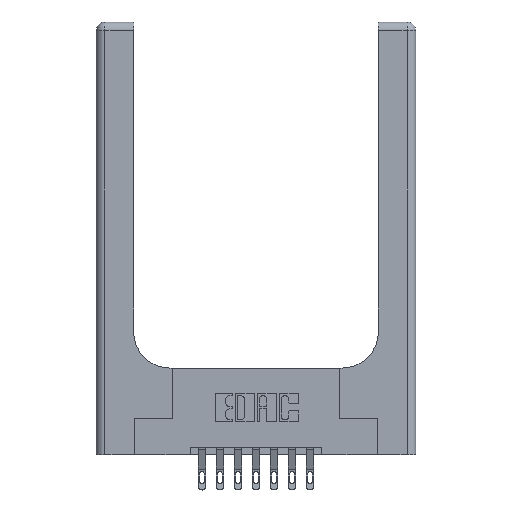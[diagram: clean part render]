
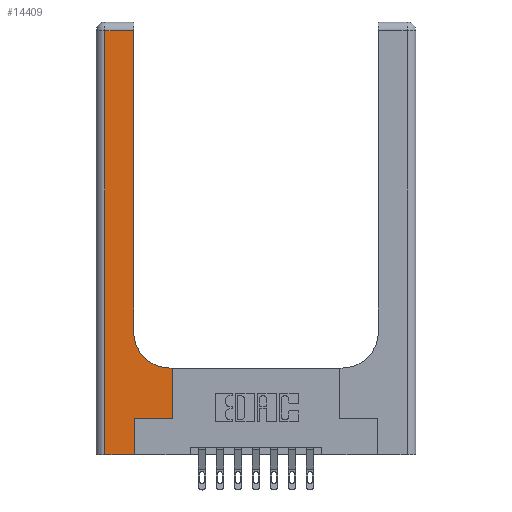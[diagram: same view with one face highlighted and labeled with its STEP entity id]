
A CAD part, top view. The second image highlights one B-rep face of the part: STEP entity #14409.
In plain terms, the highlighted planar face has unit normal (0, 0, 1).
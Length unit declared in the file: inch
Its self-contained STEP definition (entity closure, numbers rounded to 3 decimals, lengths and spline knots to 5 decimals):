
#24 = LINE ( 'NONE', #7708, #6011 ) ;
#39 = VERTEX_POINT ( 'NONE', #4736 ) ;
#306 = CARTESIAN_POINT ( 'NONE',  ( 0.528, 0.6, 0.37 ) ) ;
#439 = LINE ( 'NONE', #8988, #6055 ) ;
#632 = CARTESIAN_POINT ( 'NONE',  ( 0.265, 0., 0.37 ) ) ;
#799 = VECTOR ( 'NONE', #14047, 39.37008 ) ;
#975 = CARTESIAN_POINT ( 'NONE',  ( 0.26, 0.85, 0.37 ) ) ;
#1226 = LINE ( 'NONE', #6081, #13003 ) ;
#1489 = LINE ( 'NONE', #4487, #10914 ) ;
#1724 = EDGE_CURVE ( 'NONE', #13952, #7508, #24, .T. ) ;
#2103 = CARTESIAN_POINT ( 'NONE',  ( 0.265, 0.25, 0.37 ) ) ;
#2205 = LINE ( 'NONE', #3393, #9850 ) ;
#2329 = CIRCLE ( 'NONE', #5910, 0.25 ) ;
#2439 = ORIENTED_EDGE ( 'NONE', *, *, #13124, .T. ) ;
#2523 = DIRECTION ( 'NONE',  ( 0., 1., 0. ) ) ;
#2713 = DIRECTION ( 'NONE',  ( 0., 0., -1. ) ) ;
#3055 = EDGE_LOOP ( 'NONE', ( #2439, #11211, #13454, #9057, #4490, #14708, #9801, #5063, #7441 ) ) ;
#3193 = DIRECTION ( 'NONE',  ( 0., 1., 0. ) ) ;
#3233 = DIRECTION ( 'NONE',  ( -1., 0., 0. ) ) ;
#3324 = AXIS2_PLACEMENT_3D ( 'NONE', #4338, #7697, #5497 ) ;
#3393 = CARTESIAN_POINT ( 'NONE',  ( 0.265, 0., 0.37 ) ) ;
#3765 = VERTEX_POINT ( 'NONE', #13773 ) ;
#3940 = CARTESIAN_POINT ( 'NONE',  ( 0.528, 0.25, 0.37 ) ) ;
#4065 = VERTEX_POINT ( 'NONE', #8728 ) ;
#4338 = CARTESIAN_POINT ( 'NONE',  ( 0., 3., 0.37 ) ) ;
#4487 = CARTESIAN_POINT ( 'NONE',  ( 0.06, 3., 0.37 ) ) ;
#4490 = ORIENTED_EDGE ( 'NONE', *, *, #8910, .T. ) ;
#4506 = DIRECTION ( 'NONE',  ( 1., 0., 0. ) ) ;
#4578 = DIRECTION ( 'NONE',  ( 0., -1., 0. ) ) ;
#4736 = CARTESIAN_POINT ( 'NONE',  ( 0.06, 2.94, 0.37 ) ) ;
#5063 = ORIENTED_EDGE ( 'NONE', *, *, #5894, .T. ) ;
#5497 = DIRECTION ( 'NONE',  ( -1., 0., 0. ) ) ;
#5894 = EDGE_CURVE ( 'NONE', #7508, #4065, #14048, .T. ) ;
#5910 = AXIS2_PLACEMENT_3D ( 'NONE', #9476, #2713, #6116 ) ;
#6011 = VECTOR ( 'NONE', #3193, 39.37008 ) ;
#6044 = VERTEX_POINT ( 'NONE', #2103 ) ;
#6055 = VECTOR ( 'NONE', #3233, 39.37008 ) ;
#6081 = CARTESIAN_POINT ( 'NONE',  ( 0.26, 3., 0.37 ) ) ;
#6116 = DIRECTION ( 'NONE',  ( 1., 0., 0. ) ) ;
#7029 = CARTESIAN_POINT ( 'NONE',  ( 0.06, 0., 0.37 ) ) ;
#7037 = CARTESIAN_POINT ( 'NONE',  ( 0.265, 0.25, 0.37 ) ) ;
#7441 = ORIENTED_EDGE ( 'NONE', *, *, #7445, .T. ) ;
#7445 = EDGE_CURVE ( 'NONE', #4065, #8214, #2329, .T. ) ;
#7508 = VERTEX_POINT ( 'NONE', #306 ) ;
#7697 = DIRECTION ( 'NONE',  ( 0., 0., -1. ) ) ;
#7708 = CARTESIAN_POINT ( 'NONE',  ( 0.528, 0.25, 0.37 ) ) ;
#8103 = VERTEX_POINT ( 'NONE', #632 ) ;
#8214 = VERTEX_POINT ( 'NONE', #975 ) ;
#8281 = LINE ( 'NONE', #12607, #14424 ) ;
#8728 = CARTESIAN_POINT ( 'NONE',  ( 0.51, 0.6, 0.37 ) ) ;
#8910 = EDGE_CURVE ( 'NONE', #8103, #6044, #2205, .T. ) ;
#8988 = CARTESIAN_POINT ( 'NONE',  ( 0., 2.94, 0.37 ) ) ;
#9057 = ORIENTED_EDGE ( 'NONE', *, *, #14172, .T. ) ;
#9112 = EDGE_CURVE ( 'NONE', #39, #13638, #1489, .T. ) ;
#9241 = EDGE_CURVE ( 'NONE', #6044, #13952, #9665, .T. ) ;
#9476 = CARTESIAN_POINT ( 'NONE',  ( 0.51, 0.85, 0.37 ) ) ;
#9665 = LINE ( 'NONE', #7037, #799 ) ;
#9801 = ORIENTED_EDGE ( 'NONE', *, *, #1724, .T. ) ;
#9850 = VECTOR ( 'NONE', #9966, 39.37008 ) ;
#9966 = DIRECTION ( 'NONE',  ( 0., 1., 0. ) ) ;
#10262 = EDGE_CURVE ( 'NONE', #3765, #39, #439, .T. ) ;
#10914 = VECTOR ( 'NONE', #4578, 39.37008 ) ;
#11211 = ORIENTED_EDGE ( 'NONE', *, *, #10262, .T. ) ;
#12123 = CARTESIAN_POINT ( 'NONE',  ( 0.26, 0.6, 0.37 ) ) ;
#12594 = VECTOR ( 'NONE', #13310, 39.37008 ) ;
#12607 = CARTESIAN_POINT ( 'NONE',  ( 0., 0., 0.37 ) ) ;
#12795 = FACE_OUTER_BOUND ( 'NONE', #3055, .T. ) ;
#13003 = VECTOR ( 'NONE', #2523, 39.37008 ) ;
#13124 = EDGE_CURVE ( 'NONE', #8214, #3765, #1226, .T. ) ;
#13310 = DIRECTION ( 'NONE',  ( -1., 0., 0. ) ) ;
#13454 = ORIENTED_EDGE ( 'NONE', *, *, #9112, .T. ) ;
#13638 = VERTEX_POINT ( 'NONE', #7029 ) ;
#13773 = CARTESIAN_POINT ( 'NONE',  ( 0.26, 2.94, 0.37 ) ) ;
#13952 = VERTEX_POINT ( 'NONE', #3940 ) ;
#14047 = DIRECTION ( 'NONE',  ( 1., 0., 0. ) ) ;
#14048 = LINE ( 'NONE', #12123, #12594 ) ;
#14172 = EDGE_CURVE ( 'NONE', #13638, #8103, #8281, .T. ) ;
#14409 = ADVANCED_FACE ( 'NONE', ( #12795 ), #14728, .F. ) ;
#14424 = VECTOR ( 'NONE', #4506, 39.37008 ) ;
#14708 = ORIENTED_EDGE ( 'NONE', *, *, #9241, .T. ) ;
#14728 = PLANE ( 'NONE',  #3324 ) ;
